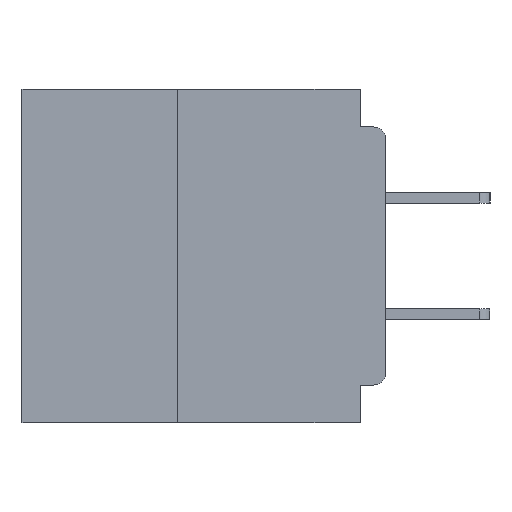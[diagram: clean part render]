
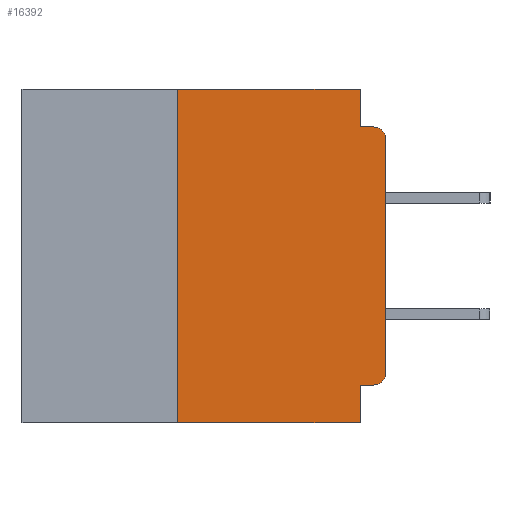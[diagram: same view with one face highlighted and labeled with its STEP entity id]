
A CAD part, left-side view. The second image highlights one B-rep face of the part: STEP entity #16392.
In plain terms, the highlighted planar face has unit normal (-1, 0, 0).
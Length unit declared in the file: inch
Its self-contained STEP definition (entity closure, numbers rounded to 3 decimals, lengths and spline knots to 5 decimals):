
#155 = CARTESIAN_POINT ( 'NONE',  ( 0., 0.015, -0.34 ) ) ;
#1500 = EDGE_CURVE ( 'NONE', #4562, #8852, #15339, .T. ) ;
#2053 = LINE ( 'NONE', #37452, #25233 ) ;
#2830 = AXIS2_PLACEMENT_3D ( 'NONE', #155, #28895, #4298 ) ;
#2958 = PLANE ( 'NONE',  #5443 ) ;
#2988 = ORIENTED_EDGE ( 'NONE', *, *, #45329, .F. ) ;
#3909 = EDGE_CURVE ( 'NONE', #36334, #13335, #2053, .T. ) ;
#4107 = VERTEX_POINT ( 'NONE', #50824 ) ;
#4150 = CARTESIAN_POINT ( 'NONE',  ( 0., 0., -0.34 ) ) ;
#4266 = CARTESIAN_POINT ( 'NONE',  ( 0., 0.015, -0.06 ) ) ;
#4277 = CARTESIAN_POINT ( 'NONE',  ( 0., 0.015, -0.355 ) ) ;
#4298 = DIRECTION ( 'NONE',  ( 0., 0., -1. ) ) ;
#4377 = CARTESIAN_POINT ( 'NONE',  ( 0., 0.437, 0. ) ) ;
#4562 = VERTEX_POINT ( 'NONE', #29346 ) ;
#5443 = AXIS2_PLACEMENT_3D ( 'NONE', #11274, #39854, #15388 ) ;
#6786 = ORIENTED_EDGE ( 'NONE', *, *, #10247, .T. ) ;
#7385 = VECTOR ( 'NONE', #18352, 39.37008 ) ;
#8392 = DIRECTION ( 'NONE',  ( 0., 0., -1. ) ) ;
#8852 = VERTEX_POINT ( 'NONE', #44866 ) ;
#9572 = VERTEX_POINT ( 'NONE', #4150 ) ;
#10247 = EDGE_CURVE ( 'NONE', #4107, #20005, #19589, .T. ) ;
#11216 = CARTESIAN_POINT ( 'NONE',  ( 0., 0., -0.355 ) ) ;
#11274 = CARTESIAN_POINT ( 'NONE',  ( 0., 0.437, 0. ) ) ;
#11445 = ORIENTED_EDGE ( 'NONE', *, *, #15623, .T. ) ;
#12851 = DIRECTION ( 'NONE',  ( 0., -1., 0. ) ) ;
#12954 = DIRECTION ( 'NONE',  ( 0., 0., 1. ) ) ;
#13335 = VERTEX_POINT ( 'NONE', #40733 ) ;
#13406 = EDGE_CURVE ( 'NONE', #13335, #46296, #21269, .T. ) ;
#13802 = EDGE_CURVE ( 'NONE', #17548, #4562, #15417, .T. ) ;
#15339 = LINE ( 'NONE', #22394, #26286 ) ;
#15340 = CARTESIAN_POINT ( 'NONE',  ( 0., 0.031, -0.045 ) ) ;
#15388 = DIRECTION ( 'NONE',  ( 0., 0., -1. ) ) ;
#15417 = LINE ( 'NONE', #11216, #49293 ) ;
#15623 = EDGE_CURVE ( 'NONE', #36334, #8852, #52221, .T. ) ;
#16392 = ADVANCED_FACE ( 'NONE', ( #20843 ), #2958, .F. ) ;
#17548 = VERTEX_POINT ( 'NONE', #4277 ) ;
#18352 = DIRECTION ( 'NONE',  ( 0., -1., 0. ) ) ;
#19589 = CIRCLE ( 'NONE', #39680, 0.015 ) ;
#20005 = VERTEX_POINT ( 'NONE', #52748 ) ;
#20843 = FACE_OUTER_BOUND ( 'NONE', #29311, .T. ) ;
#21269 = LINE ( 'NONE', #4377, #33394 ) ;
#21357 = ORIENTED_EDGE ( 'NONE', *, *, #13802, .F. ) ;
#22354 = CARTESIAN_POINT ( 'NONE',  ( 0., 0., 0. ) ) ;
#22394 = CARTESIAN_POINT ( 'NONE',  ( 0., 0.031, -0.4 ) ) ;
#22435 = EDGE_CURVE ( 'NONE', #33527, #20005, #51053, .T. ) ;
#25233 = VECTOR ( 'NONE', #12954, 39.37008 ) ;
#25592 = ORIENTED_EDGE ( 'NONE', *, *, #13406, .F. ) ;
#26286 = VECTOR ( 'NONE', #42513, 39.37008 ) ;
#26599 = CIRCLE ( 'NONE', #2830, 0.015 ) ;
#27357 = LINE ( 'NONE', #22354, #38216 ) ;
#27983 = CARTESIAN_POINT ( 'NONE',  ( 0., 0.031, 0. ) ) ;
#28895 = DIRECTION ( 'NONE',  ( -1., 0., 0. ) ) ;
#28968 = DIRECTION ( 'NONE',  ( 0., -1., 0. ) ) ;
#29311 = EDGE_LOOP ( 'NONE', ( #36079, #6786, #49093, #2988, #25592, #38482, #11445, #47766, #21357, #41792 ) ) ;
#29346 = CARTESIAN_POINT ( 'NONE',  ( 0., 0.031, -0.355 ) ) ;
#29876 = CARTESIAN_POINT ( 'NONE',  ( 0., 0.031, 0. ) ) ;
#30516 = CARTESIAN_POINT ( 'NONE',  ( 0., 0.437, -0.4 ) ) ;
#31614 = DIRECTION ( 'NONE',  ( 0., 1., 0. ) ) ;
#32824 = CARTESIAN_POINT ( 'NONE',  ( 0., 0.25, -0.4 ) ) ;
#32978 = DIRECTION ( 'NONE',  ( -1., 0., 0. ) ) ;
#33394 = VECTOR ( 'NONE', #28968, 39.37008 ) ;
#33527 = VERTEX_POINT ( 'NONE', #15340 ) ;
#36079 = ORIENTED_EDGE ( 'NONE', *, *, #45079, .T. ) ;
#36334 = VERTEX_POINT ( 'NONE', #32824 ) ;
#37452 = CARTESIAN_POINT ( 'NONE',  ( 0., 0.25, -0.4 ) ) ;
#37556 = VECTOR ( 'NONE', #40112, 39.37008 ) ;
#38216 = VECTOR ( 'NONE', #50884, 39.37008 ) ;
#38482 = ORIENTED_EDGE ( 'NONE', *, *, #3909, .F. ) ;
#38824 = LINE ( 'NONE', #27983, #37556 ) ;
#38937 = EDGE_CURVE ( 'NONE', #17548, #9572, #26599, .T. ) ;
#39680 = AXIS2_PLACEMENT_3D ( 'NONE', #4266, #32978, #8392 ) ;
#39854 = DIRECTION ( 'NONE',  ( 1., 0., 0. ) ) ;
#40112 = DIRECTION ( 'NONE',  ( 0., 0., -1. ) ) ;
#40733 = CARTESIAN_POINT ( 'NONE',  ( 0., 0.25, 0. ) ) ;
#41792 = ORIENTED_EDGE ( 'NONE', *, *, #38937, .T. ) ;
#42513 = DIRECTION ( 'NONE',  ( 0., 0., -1. ) ) ;
#44866 = CARTESIAN_POINT ( 'NONE',  ( 0., 0.031, -0.4 ) ) ;
#45079 = EDGE_CURVE ( 'NONE', #9572, #4107, #27357, .T. ) ;
#45329 = EDGE_CURVE ( 'NONE', #46296, #33527, #38824, .T. ) ;
#46296 = VERTEX_POINT ( 'NONE', #29876 ) ;
#47766 = ORIENTED_EDGE ( 'NONE', *, *, #1500, .F. ) ;
#49093 = ORIENTED_EDGE ( 'NONE', *, *, #22435, .F. ) ;
#49293 = VECTOR ( 'NONE', #31614, 39.37008 ) ;
#49463 = CARTESIAN_POINT ( 'NONE',  ( 0., 0., -0.045 ) ) ;
#49754 = VECTOR ( 'NONE', #12851, 39.37008 ) ;
#50824 = CARTESIAN_POINT ( 'NONE',  ( 0., 0., -0.06 ) ) ;
#50884 = DIRECTION ( 'NONE',  ( 0., 0., 1. ) ) ;
#51053 = LINE ( 'NONE', #49463, #49754 ) ;
#52221 = LINE ( 'NONE', #30516, #7385 ) ;
#52748 = CARTESIAN_POINT ( 'NONE',  ( 0., 0.015, -0.045 ) ) ;
